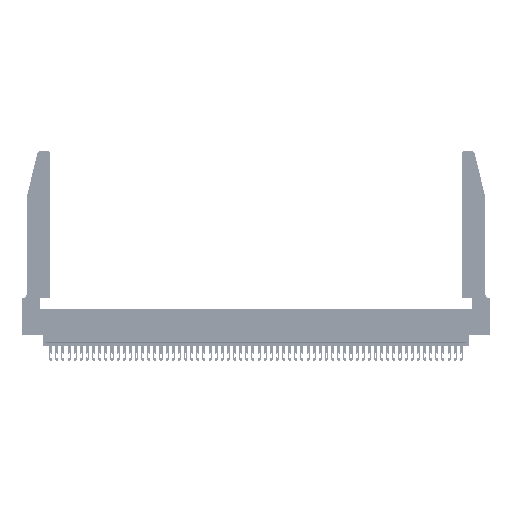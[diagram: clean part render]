
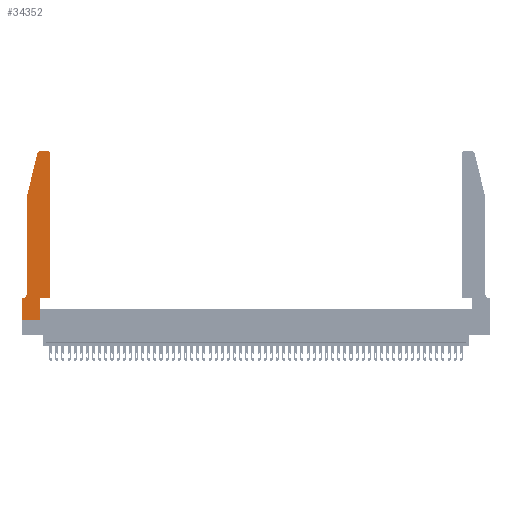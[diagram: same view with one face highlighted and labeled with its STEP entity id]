
A CAD part, top view. The second image highlights one B-rep face of the part: STEP entity #34352.
In plain terms, the highlighted planar face has unit normal (0, 0, 1).
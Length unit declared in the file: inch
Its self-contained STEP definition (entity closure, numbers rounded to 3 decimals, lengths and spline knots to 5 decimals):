
#67 = DIRECTION ( 'NONE',  ( -1., 0., 0. ) ) ;
#279 = EDGE_LOOP ( 'NONE', ( #31216, #27805, #47839, #32812, #11857, #50710, #23516, #18707, #15517, #39913, #44548, #51174 ) ) ;
#2139 = EDGE_CURVE ( 'NONE', #42866, #44700, #44702, .T. ) ;
#2203 = DIRECTION ( 'NONE',  ( 1., 0., 0. ) ) ;
#2461 = VECTOR ( 'NONE', #67, 39.37008 ) ;
#3818 = LINE ( 'NONE', #44460, #40153 ) ;
#3974 = DIRECTION ( 'NONE',  ( -1., 0., 0. ) ) ;
#4002 = CARTESIAN_POINT ( 'NONE',  ( 0.4505, 0.35, 0.37 ) ) ;
#4282 = LINE ( 'NONE', #50856, #14212 ) ;
#5213 = CIRCLE ( 'NONE', #54293, 0.03 ) ;
#5458 = VERTEX_POINT ( 'NONE', #5715 ) ;
#5715 = CARTESIAN_POINT ( 'NONE',  ( 0.4205, 2.75, 0.37 ) ) ;
#6542 = EDGE_CURVE ( 'NONE', #40249, #42866, #27798, .T. ) ;
#6701 = DIRECTION ( 'NONE',  ( 1., 0., 0. ) ) ;
#8231 = CARTESIAN_POINT ( 'NONE',  ( 0.0055, 0.42, 0.37 ) ) ;
#8277 = EDGE_CURVE ( 'NONE', #8772, #40249, #12979, .T. ) ;
#8310 = DIRECTION ( 'NONE',  ( 0., 1., 0. ) ) ;
#8772 = VERTEX_POINT ( 'NONE', #25391 ) ;
#11604 = CARTESIAN_POINT ( 'NONE',  ( 0., 0.35, 0.37 ) ) ;
#11857 = ORIENTED_EDGE ( 'NONE', *, *, #6542, .T. ) ;
#12089 = VECTOR ( 'NONE', #27507, 39.37008 ) ;
#12290 = DIRECTION ( 'NONE',  ( 0., 0., -1. ) ) ;
#12413 = VERTEX_POINT ( 'NONE', #32556 ) ;
#12932 = EDGE_CURVE ( 'NONE', #46962, #5458, #5213, .T. ) ;
#12979 = LINE ( 'NONE', #13250, #45312 ) ;
#13250 = CARTESIAN_POINT ( 'NONE',  ( 0.0755, 2., 0.37 ) ) ;
#14212 = VECTOR ( 'NONE', #3974, 39.37008 ) ;
#14565 = VERTEX_POINT ( 'NONE', #33819 ) ;
#15517 = ORIENTED_EDGE ( 'NONE', *, *, #36527, .T. ) ;
#16695 = AXIS2_PLACEMENT_3D ( 'NONE', #36281, #53026, #6701 ) ;
#17563 = EDGE_CURVE ( 'NONE', #38437, #46962, #24148, .T. ) ;
#18419 = CARTESIAN_POINT ( 'NONE',  ( 0.4505, 0.35, 0.37 ) ) ;
#18707 = ORIENTED_EDGE ( 'NONE', *, *, #31454, .T. ) ;
#18939 = EDGE_CURVE ( 'NONE', #29775, #38437, #41788, .T. ) ;
#19030 = CARTESIAN_POINT ( 'NONE',  ( 0.4505, 0.35, 0.37 ) ) ;
#19520 = LINE ( 'NONE', #27106, #36069 ) ;
#19559 = CARTESIAN_POINT ( 'NONE',  ( 0.4205, 2.72, 0.37 ) ) ;
#19753 = EDGE_CURVE ( 'NONE', #12413, #14565, #23813, .T. ) ;
#20027 = EDGE_CURVE ( 'NONE', #14565, #8772, #3818, .T. ) ;
#20631 = CARTESIAN_POINT ( 'NONE',  ( 0., 0., 0.37 ) ) ;
#22883 = DIRECTION ( 'NONE',  ( 1., 0., 0. ) ) ;
#23516 = ORIENTED_EDGE ( 'NONE', *, *, #47585, .T. ) ;
#23813 = CIRCLE ( 'NONE', #28668, 0.03 ) ;
#24148 = LINE ( 'NONE', #18419, #34749 ) ;
#24792 = DIRECTION ( 'NONE',  ( 0., 0., 1. ) ) ;
#25220 = DIRECTION ( 'NONE',  ( -1., 0., 0. ) ) ;
#25391 = CARTESIAN_POINT ( 'NONE',  ( 0.0755, 2., 0.37 ) ) ;
#27106 = CARTESIAN_POINT ( 'NONE',  ( 0., 0., 0.37 ) ) ;
#27507 = DIRECTION ( 'NONE',  ( 1., 0., 0. ) ) ;
#27798 = CIRCLE ( 'NONE', #30803, 0.07 ) ;
#27805 = ORIENTED_EDGE ( 'NONE', *, *, #19753, .T. ) ;
#27876 = DIRECTION ( 'NONE',  ( 0., 0., 1. ) ) ;
#28654 = DIRECTION ( 'NONE',  ( 1., 0., 0. ) ) ;
#28668 = AXIS2_PLACEMENT_3D ( 'NONE', #45786, #24792, #28654 ) ;
#29137 = CARTESIAN_POINT ( 'NONE',  ( 0.0755, 0.42, 0.37 ) ) ;
#29775 = VERTEX_POINT ( 'NONE', #41644 ) ;
#30056 = DIRECTION ( 'NONE',  ( 0., -1., 0. ) ) ;
#30663 = FACE_OUTER_BOUND ( 'NONE', #279, .T. ) ;
#30803 = AXIS2_PLACEMENT_3D ( 'NONE', #8231, #12290, #25220 ) ;
#31216 = ORIENTED_EDGE ( 'NONE', *, *, #49897, .T. ) ;
#31454 = EDGE_CURVE ( 'NONE', #40177, #44119, #19520, .T. ) ;
#32556 = CARTESIAN_POINT ( 'NONE',  ( 0.284, 2.75, 0.37 ) ) ;
#32812 = ORIENTED_EDGE ( 'NONE', *, *, #8277, .T. ) ;
#33819 = CARTESIAN_POINT ( 'NONE',  ( 0.25487, 2.72718, 0.37 ) ) ;
#33880 = DIRECTION ( 'NONE',  ( -0.239, -0.971, 0. ) ) ;
#34352 = ADVANCED_FACE ( 'NONE', ( #30663 ), #53382, .T. ) ;
#34749 = VECTOR ( 'NONE', #51806, 39.37008 ) ;
#36069 = VECTOR ( 'NONE', #22883, 39.37008 ) ;
#36281 = CARTESIAN_POINT ( 'NONE',  ( 0., 0.35, 0.37 ) ) ;
#36527 = EDGE_CURVE ( 'NONE', #44119, #29775, #52866, .T. ) ;
#38437 = VERTEX_POINT ( 'NONE', #4002 ) ;
#39913 = ORIENTED_EDGE ( 'NONE', *, *, #18939, .T. ) ;
#40153 = VECTOR ( 'NONE', #33880, 39.37008 ) ;
#40177 = VERTEX_POINT ( 'NONE', #20631 ) ;
#40249 = VERTEX_POINT ( 'NONE', #29137 ) ;
#40392 = CARTESIAN_POINT ( 'NONE',  ( 0.2865, 0., 0.37 ) ) ;
#41644 = CARTESIAN_POINT ( 'NONE',  ( 0.2865, 0.35, 0.37 ) ) ;
#41782 = CARTESIAN_POINT ( 'NONE',  ( 0.0055, 0.35, 0.37 ) ) ;
#41788 = LINE ( 'NONE', #19030, #12089 ) ;
#41872 = CARTESIAN_POINT ( 'NONE',  ( 0.2865, 0.35, 0.37 ) ) ;
#42866 = VERTEX_POINT ( 'NONE', #41782 ) ;
#44119 = VERTEX_POINT ( 'NONE', #40392 ) ;
#44213 = CARTESIAN_POINT ( 'NONE',  ( 0.4505, 2.72, 0.37 ) ) ;
#44390 = DIRECTION ( 'NONE',  ( 0., -1., 0. ) ) ;
#44460 = CARTESIAN_POINT ( 'NONE',  ( 0.0755, 2., 0.37 ) ) ;
#44548 = ORIENTED_EDGE ( 'NONE', *, *, #17563, .T. ) ;
#44700 = VERTEX_POINT ( 'NONE', #11604 ) ;
#44702 = LINE ( 'NONE', #51031, #2461 ) ;
#45312 = VECTOR ( 'NONE', #30056, 39.37008 ) ;
#45786 = CARTESIAN_POINT ( 'NONE',  ( 0.284, 2.72, 0.37 ) ) ;
#46784 = LINE ( 'NONE', #52359, #48069 ) ;
#46962 = VERTEX_POINT ( 'NONE', #44213 ) ;
#47548 = VECTOR ( 'NONE', #8310, 39.37008 ) ;
#47585 = EDGE_CURVE ( 'NONE', #44700, #40177, #46784, .T. ) ;
#47839 = ORIENTED_EDGE ( 'NONE', *, *, #20027, .T. ) ;
#48069 = VECTOR ( 'NONE', #44390, 39.37008 ) ;
#49897 = EDGE_CURVE ( 'NONE', #5458, #12413, #4282, .T. ) ;
#50710 = ORIENTED_EDGE ( 'NONE', *, *, #2139, .T. ) ;
#50856 = CARTESIAN_POINT ( 'NONE',  ( 0.2605, 2.75, 0.37 ) ) ;
#51031 = CARTESIAN_POINT ( 'NONE',  ( 0.0755, 0.35, 0.37 ) ) ;
#51174 = ORIENTED_EDGE ( 'NONE', *, *, #12932, .T. ) ;
#51806 = DIRECTION ( 'NONE',  ( 0., 1., 0. ) ) ;
#52359 = CARTESIAN_POINT ( 'NONE',  ( 0., 0., 0.37 ) ) ;
#52866 = LINE ( 'NONE', #41872, #47548 ) ;
#53026 = DIRECTION ( 'NONE',  ( 0., 0., 1. ) ) ;
#53382 = PLANE ( 'NONE',  #16695 ) ;
#54293 = AXIS2_PLACEMENT_3D ( 'NONE', #19559, #27876, #2203 ) ;
